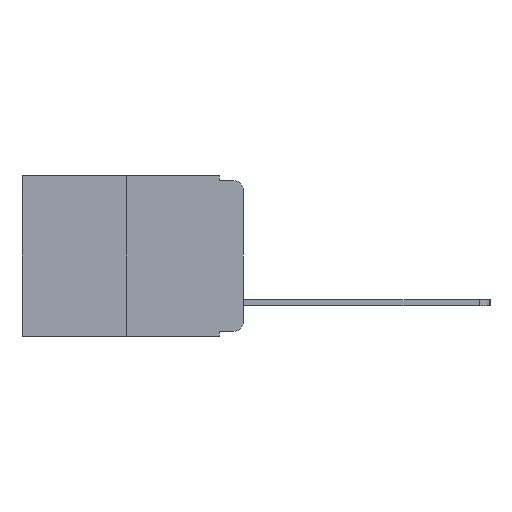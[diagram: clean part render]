
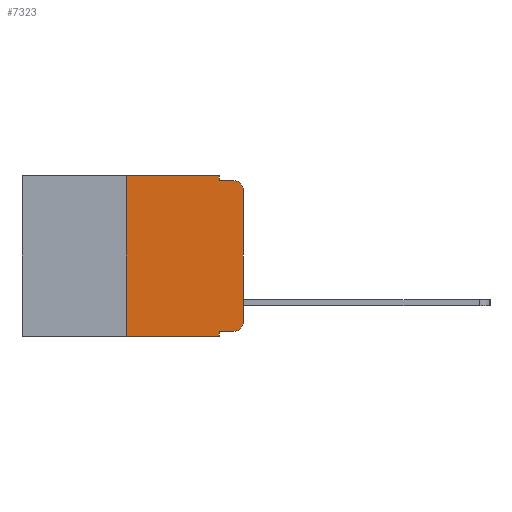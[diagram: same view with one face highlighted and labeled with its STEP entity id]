
A CAD part, left-side view. The second image highlights one B-rep face of the part: STEP entity #7323.
In plain terms, the highlighted planar face has unit normal (-1, 0, 0).
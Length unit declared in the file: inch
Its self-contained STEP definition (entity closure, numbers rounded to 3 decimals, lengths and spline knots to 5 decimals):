
#17 = CARTESIAN_POINT ( 'NONE',  ( 0., 0.473, 0. ) ) ;
#58 = CARTESIAN_POINT ( 'NONE',  ( 0., 0.051, 0. ) ) ;
#161 = DIRECTION ( 'NONE',  ( 0., -1., 0. ) ) ;
#292 = CARTESIAN_POINT ( 'NONE',  ( 0., 0., 0. ) ) ;
#327 = EDGE_LOOP ( 'NONE', ( #9673, #10143, #18474, #8708, #10640, #12493, #14506, #16721, #14958, #6444 ) ) ;
#330 = CARTESIAN_POINT ( 'NONE',  ( 0., 0.02, -0.01 ) ) ;
#856 = CARTESIAN_POINT ( 'NONE',  ( 0., 0.02, -0.313 ) ) ;
#968 = CARTESIAN_POINT ( 'NONE',  ( 0., 0.051, -0.333 ) ) ;
#1003 = CARTESIAN_POINT ( 'NONE',  ( 0., 0.25, -0.343 ) ) ;
#1388 = FACE_OUTER_BOUND ( 'NONE', #327, .T. ) ;
#1862 = EDGE_CURVE ( 'NONE', #14166, #15171, #10699, .T. ) ;
#2051 = CARTESIAN_POINT ( 'NONE',  ( 0., 0.051, -0.343 ) ) ;
#2353 = EDGE_CURVE ( 'NONE', #3381, #15125, #18200, .T. ) ;
#2416 = AXIS2_PLACEMENT_3D ( 'NONE', #856, #7767, #17376 ) ;
#3381 = VERTEX_POINT ( 'NONE', #3392 ) ;
#3392 = CARTESIAN_POINT ( 'NONE',  ( 0., 0.02, -0.333 ) ) ;
#3526 = VECTOR ( 'NONE', #9638, 39.37008 ) ;
#3737 = DIRECTION ( 'NONE',  ( -1., 0., 0. ) ) ;
#3912 = VERTEX_POINT ( 'NONE', #10864 ) ;
#4018 = VERTEX_POINT ( 'NONE', #17638 ) ;
#4694 = CARTESIAN_POINT ( 'NONE',  ( 0., 0.25, 0. ) ) ;
#5183 = EDGE_CURVE ( 'NONE', #7964, #6011, #11920, .T. ) ;
#5243 = EDGE_CURVE ( 'NONE', #7939, #7964, #18120, .T. ) ;
#5412 = VECTOR ( 'NONE', #7362, 39.37008 ) ;
#5507 = EDGE_CURVE ( 'NONE', #15125, #4018, #17453, .T. ) ;
#5663 = VECTOR ( 'NONE', #15485, 39.37008 ) ;
#6011 = VERTEX_POINT ( 'NONE', #14711 ) ;
#6176 = EDGE_CURVE ( 'NONE', #7939, #15171, #12750, .T. ) ;
#6444 = ORIENTED_EDGE ( 'NONE', *, *, #2353, .T. ) ;
#6838 = PLANE ( 'NONE',  #11663 ) ;
#6844 = CARTESIAN_POINT ( 'NONE',  ( 0., 0.473, 0. ) ) ;
#7323 = ADVANCED_FACE ( 'NONE', ( #1388 ), #6838, .F. ) ;
#7362 = DIRECTION ( 'NONE',  ( 0., -1., 0. ) ) ;
#7767 = DIRECTION ( 'NONE',  ( -1., 0., 0. ) ) ;
#7939 = VERTEX_POINT ( 'NONE', #1003 ) ;
#7964 = VERTEX_POINT ( 'NONE', #12596 ) ;
#8708 = ORIENTED_EDGE ( 'NONE', *, *, #15033, .F. ) ;
#9305 = CARTESIAN_POINT ( 'NONE',  ( 0., 0.051, 0. ) ) ;
#9334 = EDGE_CURVE ( 'NONE', #14166, #3381, #17347, .T. ) ;
#9638 = DIRECTION ( 'NONE',  ( 0., -1., 0. ) ) ;
#9673 = ORIENTED_EDGE ( 'NONE', *, *, #5507, .T. ) ;
#9872 = LINE ( 'NONE', #58, #5663 ) ;
#10143 = ORIENTED_EDGE ( 'NONE', *, *, #14444, .T. ) ;
#10640 = ORIENTED_EDGE ( 'NONE', *, *, #5183, .F. ) ;
#10699 = LINE ( 'NONE', #9305, #14120 ) ;
#10864 = CARTESIAN_POINT ( 'NONE',  ( 0., 0.051, -0.01 ) ) ;
#10962 = VECTOR ( 'NONE', #13908, 39.37008 ) ;
#11175 = EDGE_CURVE ( 'NONE', #3912, #12250, #15046, .T. ) ;
#11220 = VECTOR ( 'NONE', #161, 39.37008 ) ;
#11251 = DIRECTION ( 'NONE',  ( 0., 0., 1. ) ) ;
#11314 = CARTESIAN_POINT ( 'NONE',  ( 0., 0.051, -0.01 ) ) ;
#11421 = CARTESIAN_POINT ( 'NONE',  ( 0., 0., -0.313 ) ) ;
#11663 = AXIS2_PLACEMENT_3D ( 'NONE', #6844, #19046, #18867 ) ;
#11920 = LINE ( 'NONE', #17, #3526 ) ;
#12250 = VERTEX_POINT ( 'NONE', #330 ) ;
#12305 = VECTOR ( 'NONE', #14752, 39.37008 ) ;
#12493 = ORIENTED_EDGE ( 'NONE', *, *, #5243, .F. ) ;
#12596 = CARTESIAN_POINT ( 'NONE',  ( 0., 0.25, 0. ) ) ;
#12750 = LINE ( 'NONE', #14951, #12305 ) ;
#13048 = AXIS2_PLACEMENT_3D ( 'NONE', #13085, #3737, #14521 ) ;
#13085 = CARTESIAN_POINT ( 'NONE',  ( 0., 0.02, -0.03 ) ) ;
#13234 = VECTOR ( 'NONE', #11251, 39.37008 ) ;
#13908 = DIRECTION ( 'NONE',  ( 0., 0., 1. ) ) ;
#14120 = VECTOR ( 'NONE', #15649, 39.37008 ) ;
#14166 = VERTEX_POINT ( 'NONE', #18163 ) ;
#14444 = EDGE_CURVE ( 'NONE', #4018, #12250, #15157, .T. ) ;
#14506 = ORIENTED_EDGE ( 'NONE', *, *, #6176, .T. ) ;
#14521 = DIRECTION ( 'NONE',  ( 0., 0., -1. ) ) ;
#14711 = CARTESIAN_POINT ( 'NONE',  ( 0., 0.051, 0. ) ) ;
#14752 = DIRECTION ( 'NONE',  ( 0., -1., 0. ) ) ;
#14951 = CARTESIAN_POINT ( 'NONE',  ( 0., 0.473, -0.343 ) ) ;
#14958 = ORIENTED_EDGE ( 'NONE', *, *, #9334, .T. ) ;
#15033 = EDGE_CURVE ( 'NONE', #6011, #3912, #9872, .T. ) ;
#15046 = LINE ( 'NONE', #11314, #11220 ) ;
#15125 = VERTEX_POINT ( 'NONE', #11421 ) ;
#15157 = CIRCLE ( 'NONE', #13048, 0.02 ) ;
#15171 = VERTEX_POINT ( 'NONE', #2051 ) ;
#15485 = DIRECTION ( 'NONE',  ( 0., 0., -1. ) ) ;
#15649 = DIRECTION ( 'NONE',  ( 0., 0., -1. ) ) ;
#16721 = ORIENTED_EDGE ( 'NONE', *, *, #1862, .F. ) ;
#17347 = LINE ( 'NONE', #968, #5412 ) ;
#17376 = DIRECTION ( 'NONE',  ( 0., 0., -1. ) ) ;
#17453 = LINE ( 'NONE', #292, #13234 ) ;
#17638 = CARTESIAN_POINT ( 'NONE',  ( 0., 0., -0.03 ) ) ;
#18120 = LINE ( 'NONE', #4694, #10962 ) ;
#18163 = CARTESIAN_POINT ( 'NONE',  ( 0., 0.051, -0.333 ) ) ;
#18200 = CIRCLE ( 'NONE', #2416, 0.02 ) ;
#18474 = ORIENTED_EDGE ( 'NONE', *, *, #11175, .F. ) ;
#18867 = DIRECTION ( 'NONE',  ( 0., 0., -1. ) ) ;
#19046 = DIRECTION ( 'NONE',  ( 1., 0., 0. ) ) ;
